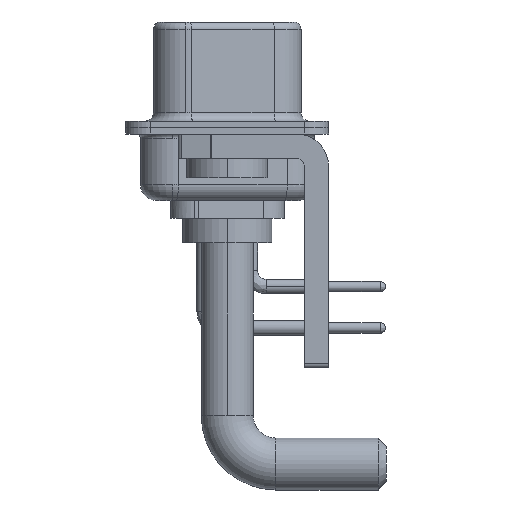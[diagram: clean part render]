
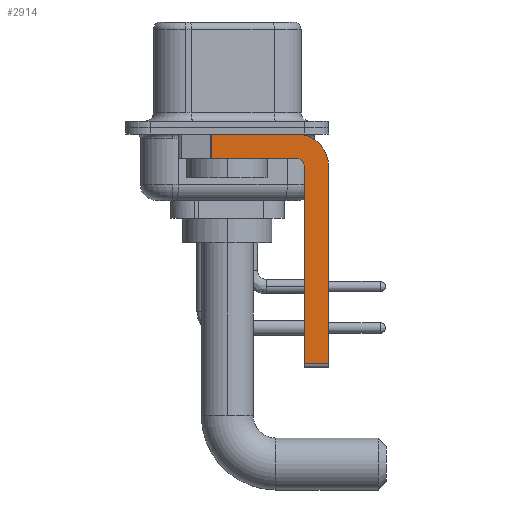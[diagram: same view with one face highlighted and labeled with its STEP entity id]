
A CAD part, left-side view. The second image highlights one B-rep face of the part: STEP entity #2914.
In plain terms, the highlighted planar face has unit normal (-1, 0, 0).
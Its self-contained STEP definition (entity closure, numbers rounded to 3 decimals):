
#80 = CARTESIAN_POINT ( 'NONE',  ( -2.9, -4.75, -2.4 ) ) ;
#90 = CARTESIAN_POINT ( 'NONE',  ( -2.9, -4.25, -1.9 ) ) ;
#94 = EDGE_CURVE ( 'NONE', #167, #2792, #4163, .T. ) ;
#167 = VERTEX_POINT ( 'NONE', #11781 ) ;
#542 = CARTESIAN_POINT ( 'NONE',  ( -2.9, -4.25, -2.4 ) ) ;
#1065 = DIRECTION ( 'NONE',  ( 0., -1., 0. ) ) ;
#1184 = CARTESIAN_POINT ( 'NONE',  ( -2.9, -4.25, -14.55 ) ) ;
#1499 = AXIS2_PLACEMENT_3D ( 'NONE', #542, #7770, #14999 ) ;
#2038 = CARTESIAN_POINT ( 'NONE',  ( -2.9, 3., -0.4 ) ) ;
#2406 = DIRECTION ( 'NONE',  ( 0., 0., -1. ) ) ;
#2792 = VERTEX_POINT ( 'NONE', #18632 ) ;
#2799 = EDGE_CURVE ( 'NONE', #17170, #4603, #5838, .T. ) ;
#2821 = CARTESIAN_POINT ( 'NONE',  ( -2.9, -4.25, -2.4 ) ) ;
#2914 = ADVANCED_FACE ( 'NONE', ( #15450 ), #17697, .F. ) ;
#3015 = VECTOR ( 'NONE', #11624, 1000. ) ;
#3853 = EDGE_CURVE ( 'NONE', #21387, #17170, #16517, .T. ) ;
#4163 = LINE ( 'NONE', #11429, #17140 ) ;
#4362 = CARTESIAN_POINT ( 'NONE',  ( -2.9, -4.75, -14.8 ) ) ;
#4533 = DIRECTION ( 'NONE',  ( 0., 0., -1. ) ) ;
#4603 = VERTEX_POINT ( 'NONE', #16117 ) ;
#4684 = VERTEX_POINT ( 'NONE', #21436 ) ;
#4723 = VECTOR ( 'NONE', #2406, 1000. ) ;
#5008 = CARTESIAN_POINT ( 'NONE',  ( -2.9, -4.25, -2.4 ) ) ;
#5838 = LINE ( 'NONE', #22302, #4723 ) ;
#5843 = EDGE_CURVE ( 'NONE', #18897, #4603, #23078, .T. ) ;
#6680 = DIRECTION ( 'NONE',  ( 1., 0., 0. ) ) ;
#7057 = CARTESIAN_POINT ( 'NONE',  ( -2.9, -6.25, -2.4 ) ) ;
#7257 = ORIENTED_EDGE ( 'NONE', *, *, #2799, .F. ) ;
#7303 = VECTOR ( 'NONE', #16730, 1000. ) ;
#7770 = DIRECTION ( 'NONE',  ( -1., 0., 0. ) ) ;
#8488 = EDGE_CURVE ( 'NONE', #18897, #19071, #14829, .T. ) ;
#8543 = ORIENTED_EDGE ( 'NONE', *, *, #3853, .F. ) ;
#8977 = AXIS2_PLACEMENT_3D ( 'NONE', #2821, #13868, #9824 ) ;
#9824 = DIRECTION ( 'NONE',  ( 0., 0., -1. ) ) ;
#10179 = EDGE_CURVE ( 'NONE', #19071, #4684, #17380, .T. ) ;
#10407 = CARTESIAN_POINT ( 'NONE',  ( -2.9, -4.25, -0.4 ) ) ;
#10885 = LINE ( 'NONE', #90, #16868 ) ;
#11420 = ORIENTED_EDGE ( 'NONE', *, *, #22547, .F. ) ;
#11429 = CARTESIAN_POINT ( 'NONE',  ( -2.9, 0.978, -1.9 ) ) ;
#11462 = ORIENTED_EDGE ( 'NONE', *, *, #94, .T. ) ;
#11624 = DIRECTION ( 'NONE',  ( 0., 0., 1. ) ) ;
#11781 = CARTESIAN_POINT ( 'NONE',  ( -2.9, 0.978, -0.4 ) ) ;
#12782 = VECTOR ( 'NONE', #1065, 1000. ) ;
#13868 = DIRECTION ( 'NONE',  ( 1., 0., 0. ) ) ;
#14600 = AXIS2_PLACEMENT_3D ( 'NONE', #5008, #6680, #4533 ) ;
#14661 = DIRECTION ( 'NONE',  ( 0., 1., 0. ) ) ;
#14829 = LINE ( 'NONE', #4362, #3015 ) ;
#14999 = DIRECTION ( 'NONE',  ( 0., 0., 1. ) ) ;
#15450 = FACE_OUTER_BOUND ( 'NONE', #17087, .T. ) ;
#16039 = ORIENTED_EDGE ( 'NONE', *, *, #18344, .F. ) ;
#16117 = CARTESIAN_POINT ( 'NONE',  ( -2.9, -6.25, -14.55 ) ) ;
#16517 = CIRCLE ( 'NONE', #8977, 2. ) ;
#16730 = DIRECTION ( 'NONE',  ( 0., -1., 0. ) ) ;
#16868 = VECTOR ( 'NONE', #14661, 1000. ) ;
#17087 = EDGE_LOOP ( 'NONE', ( #16039, #11462, #11420, #23076, #20475, #18969, #7257, #8543 ) ) ;
#17140 = VECTOR ( 'NONE', #18620, 1000. ) ;
#17170 = VERTEX_POINT ( 'NONE', #7057 ) ;
#17380 = CIRCLE ( 'NONE', #1499, 0.5 ) ;
#17697 = PLANE ( 'NONE',  #14600 ) ;
#18265 = LINE ( 'NONE', #2038, #7303 ) ;
#18344 = EDGE_CURVE ( 'NONE', #167, #21387, #18265, .T. ) ;
#18620 = DIRECTION ( 'NONE',  ( 0., 0., -1. ) ) ;
#18632 = CARTESIAN_POINT ( 'NONE',  ( -2.9, 0.978, -1.9 ) ) ;
#18897 = VERTEX_POINT ( 'NONE', #22677 ) ;
#18969 = ORIENTED_EDGE ( 'NONE', *, *, #5843, .T. ) ;
#19071 = VERTEX_POINT ( 'NONE', #80 ) ;
#20475 = ORIENTED_EDGE ( 'NONE', *, *, #8488, .F. ) ;
#21387 = VERTEX_POINT ( 'NONE', #10407 ) ;
#21436 = CARTESIAN_POINT ( 'NONE',  ( -2.9, -4.25, -1.9 ) ) ;
#22302 = CARTESIAN_POINT ( 'NONE',  ( -2.9, -6.25, -2.4 ) ) ;
#22547 = EDGE_CURVE ( 'NONE', #4684, #2792, #10885, .T. ) ;
#22677 = CARTESIAN_POINT ( 'NONE',  ( -2.9, -4.75, -14.55 ) ) ;
#23076 = ORIENTED_EDGE ( 'NONE', *, *, #10179, .F. ) ;
#23078 = LINE ( 'NONE', #1184, #12782 ) ;
